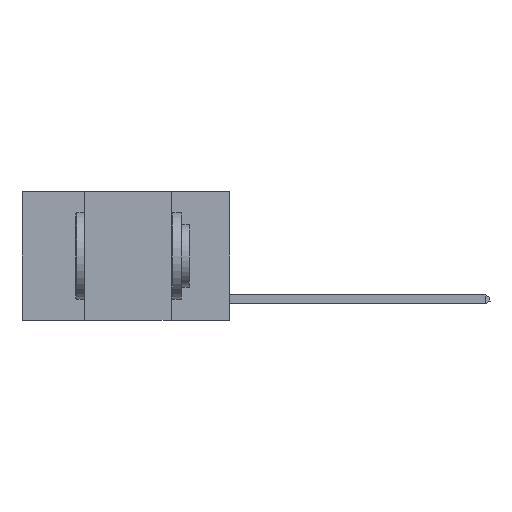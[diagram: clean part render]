
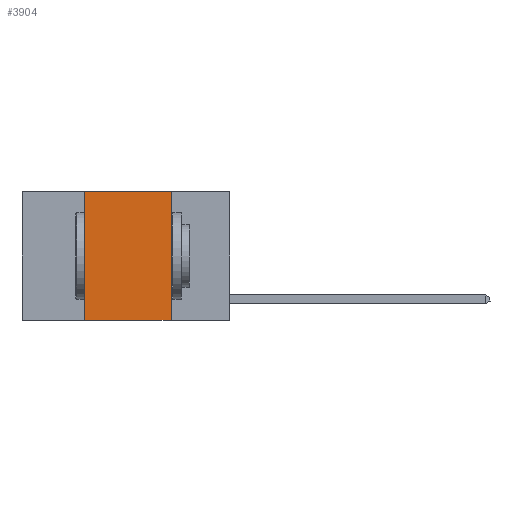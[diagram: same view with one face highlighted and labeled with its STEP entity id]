
A CAD part, left-side view. The second image highlights one B-rep face of the part: STEP entity #3904.
In plain terms, the highlighted planar face has unit normal (-1, 0, 0).
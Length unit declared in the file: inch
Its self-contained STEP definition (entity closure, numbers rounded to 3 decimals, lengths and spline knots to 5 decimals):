
#2517 = DIRECTION ( 'NONE',  ( 0., -1., 0. ) ) ;
#3904 = ADVANCED_FACE ( 'NONE', ( #22870 ), #9655, .F. ) ;
#4400 = CARTESIAN_POINT ( 'NONE',  ( 0., 0.17, 0. ) ) ;
#5294 = DIRECTION ( 'NONE',  ( 1., 0., 0. ) ) ;
#5474 = LINE ( 'NONE', #22611, #23292 ) ;
#6847 = CARTESIAN_POINT ( 'NONE',  ( 0., 0.42, 0. ) ) ;
#7824 = EDGE_LOOP ( 'NONE', ( #23860, #19351, #8113, #14065 ) ) ;
#8113 = ORIENTED_EDGE ( 'NONE', *, *, #21796, .F. ) ;
#9191 = CARTESIAN_POINT ( 'NONE',  ( 0., 0.42, 0. ) ) ;
#9239 = CARTESIAN_POINT ( 'NONE',  ( 0., 0.42, -0.37 ) ) ;
#9655 = PLANE ( 'NONE',  #9959 ) ;
#9959 = AXIS2_PLACEMENT_3D ( 'NONE', #14177, #5294, #20929 ) ;
#10498 = VECTOR ( 'NONE', #11027, 39.37008 ) ;
#11027 = DIRECTION ( 'NONE',  ( 0., -1., 0. ) ) ;
#11188 = CARTESIAN_POINT ( 'NONE',  ( 0., 0.17, -0.37 ) ) ;
#12439 = VERTEX_POINT ( 'NONE', #6847 ) ;
#12552 = VECTOR ( 'NONE', #13356, 39.37008 ) ;
#12771 = CARTESIAN_POINT ( 'NONE',  ( 0., 0.17, 0. ) ) ;
#12948 = EDGE_CURVE ( 'NONE', #27428, #12992, #18510, .T. ) ;
#12992 = VERTEX_POINT ( 'NONE', #11188 ) ;
#13266 = VECTOR ( 'NONE', #15989, 39.37008 ) ;
#13356 = DIRECTION ( 'NONE',  ( 0., 0., -1. ) ) ;
#14065 = ORIENTED_EDGE ( 'NONE', *, *, #15258, .T. ) ;
#14177 = CARTESIAN_POINT ( 'NONE',  ( 0., 0.6, 0. ) ) ;
#15258 = EDGE_CURVE ( 'NONE', #18497, #12992, #5474, .T. ) ;
#15989 = DIRECTION ( 'NONE',  ( 0., 0., 1. ) ) ;
#18497 = VERTEX_POINT ( 'NONE', #9239 ) ;
#18510 = LINE ( 'NONE', #4400, #12552 ) ;
#19248 = LINE ( 'NONE', #9191, #13266 ) ;
#19351 = ORIENTED_EDGE ( 'NONE', *, *, #20402, .F. ) ;
#19977 = CARTESIAN_POINT ( 'NONE',  ( 0., 0.6, 0. ) ) ;
#20402 = EDGE_CURVE ( 'NONE', #12439, #27428, #28273, .T. ) ;
#20929 = DIRECTION ( 'NONE',  ( 0., 0., -1. ) ) ;
#21796 = EDGE_CURVE ( 'NONE', #18497, #12439, #19248, .T. ) ;
#22611 = CARTESIAN_POINT ( 'NONE',  ( 0., 0.6, -0.37 ) ) ;
#22870 = FACE_OUTER_BOUND ( 'NONE', #7824, .T. ) ;
#23292 = VECTOR ( 'NONE', #2517, 39.37008 ) ;
#23860 = ORIENTED_EDGE ( 'NONE', *, *, #12948, .F. ) ;
#27428 = VERTEX_POINT ( 'NONE', #12771 ) ;
#28273 = LINE ( 'NONE', #19977, #10498 ) ;
